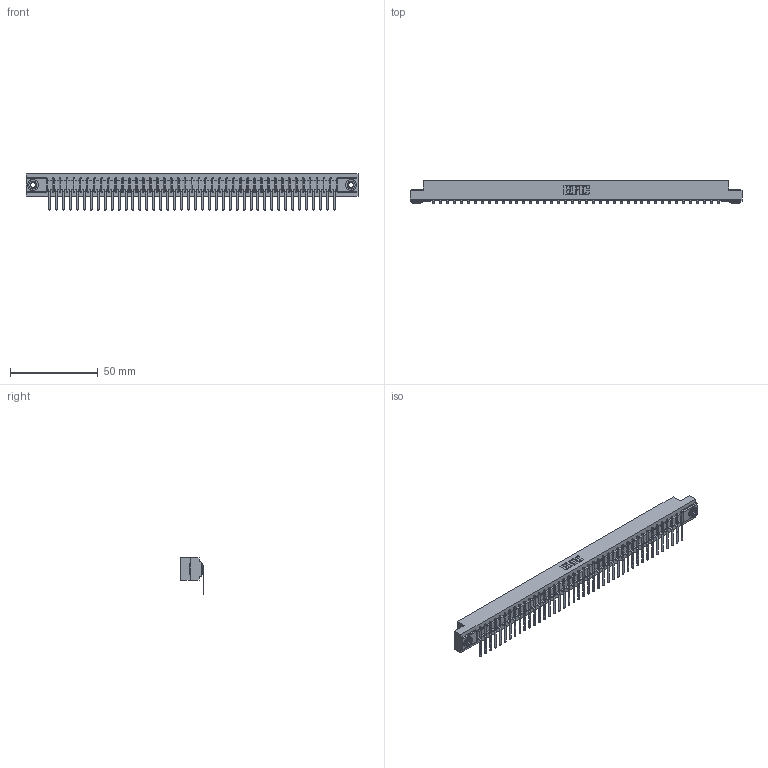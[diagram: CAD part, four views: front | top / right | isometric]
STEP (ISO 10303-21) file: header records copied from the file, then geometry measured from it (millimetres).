
FILE_DESCRIPTION (( 'STEP AP203' ), '1' );
FILE_NAME ('307-042-557-103.STEP', '2018-08-05T17:50:06', ( '' ), ( '' ), 'SwSTEP 2.0', 'SolidWorks 2016', '' );
FILE_SCHEMA (( 'CONFIG_CONTROL_DESIGN' ));
Length unit declared in the file: inch
Products named in the file (4): 345-250-002_345-250-002-102; 307-042-557-103; 307 Part_.156 Dia Mounting Holes; 307-290-002_557
Assembly tree (45 placements, depth 2):
  307-042-557-103
    307 Part_.156 Dia Mounting Holes
    307-290-002_557  x42
    345-250-002_345-250-002-102  x2
Bounding box: 189.43 x 13.36 x 20.66 mm (x, y, z)
Volume: 20386.4 mm3; surface area: 26618.8 mm2
Topology: 45 solids, 45 shells, 3489 faces, 10683 edges, 7002 vertices
Faces by surface type: plane 2068, cylinder 1327, sphere 86, cone 8
Entity records: 37925 total; most frequent: CARTESIAN_POINT 6377, ORIENTED_EDGE 6358, DIRECTION 6211, EDGE_CURVE 3179, LINE 2427, VECTOR 2427, VERTEX_POINT 2058, AXIS2_PLACEMENT_3D 1892
